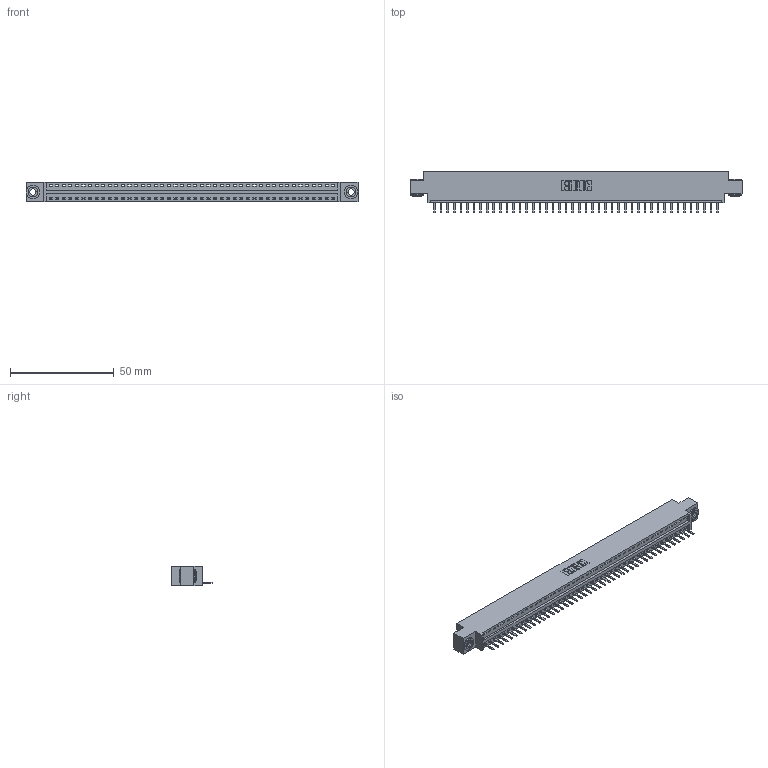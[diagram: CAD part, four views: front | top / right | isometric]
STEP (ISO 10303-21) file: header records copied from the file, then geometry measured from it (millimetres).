
FILE_DESCRIPTION (( 'STEP AP203' ), '1' );
FILE_NAME ('396-044-520-603.STEP', '2019-10-27T23:17:39', ( '' ), ( '' ), 'SwSTEP 2.0', 'SolidWorks 2016', '' );
FILE_SCHEMA (( 'CONFIG_CONTROL_DESIGN' ));
Length unit declared in the file: inch
Products named in the file (4): 396-044-520-603; 345-250-002_345-250-002-102; 346 Part_0.170 Offset - 0.156 Dia-TH; 345-292-001_345-293-120
Assembly tree (47 placements, depth 2):
  396-044-520-603
    346 Part_0.170 Offset - 0.156 Dia-TH
    345-292-001_345-293-120  x44
    345-250-002_345-250-002-102  x2
Bounding box: 160.27 x 20.02 x 9.4 mm (x, y, z)
Volume: 15093.8 mm3; surface area: 18843.9 mm2
Topology: 47 solids, 47 shells, 2892 faces, 8513 edges, 5554 vertices
Faces by surface type: plane 1938, cylinder 946, cone 8
Entity records: 27934 total; most frequent: CARTESIAN_POINT 4779, ORIENTED_EDGE 4738, DIRECTION 4231, EDGE_CURVE 2369, VECTOR 2033, LINE 2033, VERTEX_POINT 1574, AXIS2_PLACEMENT_3D 1099
